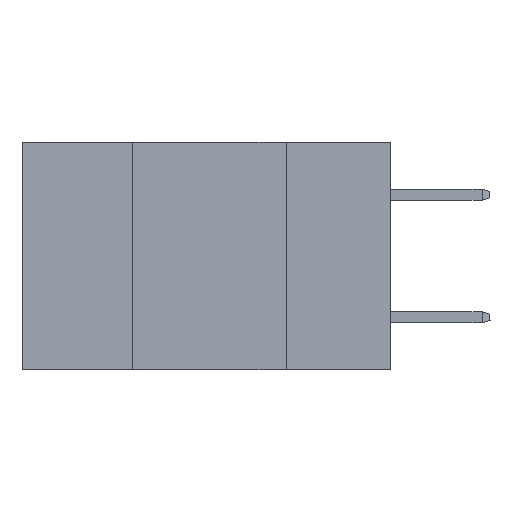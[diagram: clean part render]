
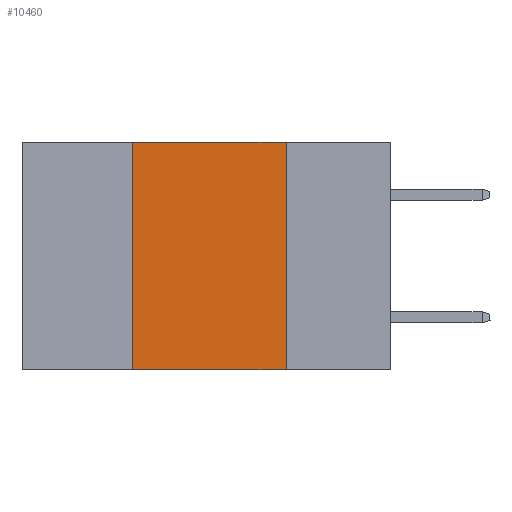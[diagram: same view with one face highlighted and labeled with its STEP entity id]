
A CAD part, left-side view. The second image highlights one B-rep face of the part: STEP entity #10460.
In plain terms, the highlighted planar face has unit normal (-1, 0, 0).
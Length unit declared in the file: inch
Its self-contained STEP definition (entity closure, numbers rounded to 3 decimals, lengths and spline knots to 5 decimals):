
#640 = CARTESIAN_POINT ( 'NONE',  ( 0., 0.6, -0.37 ) ) ;
#650 = EDGE_CURVE ( 'NONE', #4105, #13958, #9030, .T. ) ;
#963 = EDGE_CURVE ( 'NONE', #13958, #3943, #14695, .T. ) ;
#1072 = DIRECTION ( 'NONE',  ( 0., -1., 0. ) ) ;
#1235 = CARTESIAN_POINT ( 'NONE',  ( 0., 0.6, 0. ) ) ;
#2109 = CARTESIAN_POINT ( 'NONE',  ( 0., 0.6, 0. ) ) ;
#2661 = LINE ( 'NONE', #16177, #9623 ) ;
#2712 = CARTESIAN_POINT ( 'NONE',  ( 0., 0.17, -0.37 ) ) ;
#3750 = ORIENTED_EDGE ( 'NONE', *, *, #650, .F. ) ;
#3943 = VERTEX_POINT ( 'NONE', #2712 ) ;
#4105 = VERTEX_POINT ( 'NONE', #6254 ) ;
#4217 = VECTOR ( 'NONE', #7673, 39.37008 ) ;
#4671 = LINE ( 'NONE', #640, #4217 ) ;
#5398 = DIRECTION ( 'NONE',  ( 0., 0., 1. ) ) ;
#5913 = AXIS2_PLACEMENT_3D ( 'NONE', #2109, #7769, #17030 ) ;
#6254 = CARTESIAN_POINT ( 'NONE',  ( 0., 0.42, 0. ) ) ;
#6378 = CARTESIAN_POINT ( 'NONE',  ( 0., 0.42, -0.37 ) ) ;
#7092 = EDGE_CURVE ( 'NONE', #7806, #3943, #4671, .T. ) ;
#7120 = CARTESIAN_POINT ( 'NONE',  ( 0., 0.17, 0. ) ) ;
#7673 = DIRECTION ( 'NONE',  ( 0., -1., 0. ) ) ;
#7769 = DIRECTION ( 'NONE',  ( 1., 0., 0. ) ) ;
#7806 = VERTEX_POINT ( 'NONE', #6378 ) ;
#9030 = LINE ( 'NONE', #1235, #12219 ) ;
#9623 = VECTOR ( 'NONE', #5398, 39.37008 ) ;
#10238 = ORIENTED_EDGE ( 'NONE', *, *, #15795, .F. ) ;
#10460 = ADVANCED_FACE ( 'NONE', ( #12291 ), #11790, .F. ) ;
#11132 = VECTOR ( 'NONE', #11960, 39.37008 ) ;
#11790 = PLANE ( 'NONE',  #5913 ) ;
#11960 = DIRECTION ( 'NONE',  ( 0., 0., -1. ) ) ;
#12219 = VECTOR ( 'NONE', #1072, 39.37008 ) ;
#12291 = FACE_OUTER_BOUND ( 'NONE', #13278, .T. ) ;
#12933 = CARTESIAN_POINT ( 'NONE',  ( 0., 0.17, 0. ) ) ;
#13278 = EDGE_LOOP ( 'NONE', ( #14951, #3750, #10238, #13999 ) ) ;
#13958 = VERTEX_POINT ( 'NONE', #12933 ) ;
#13999 = ORIENTED_EDGE ( 'NONE', *, *, #7092, .T. ) ;
#14695 = LINE ( 'NONE', #7120, #11132 ) ;
#14951 = ORIENTED_EDGE ( 'NONE', *, *, #963, .F. ) ;
#15795 = EDGE_CURVE ( 'NONE', #7806, #4105, #2661, .T. ) ;
#16177 = CARTESIAN_POINT ( 'NONE',  ( 0., 0.42, 0. ) ) ;
#17030 = DIRECTION ( 'NONE',  ( 0., 0., -1. ) ) ;
